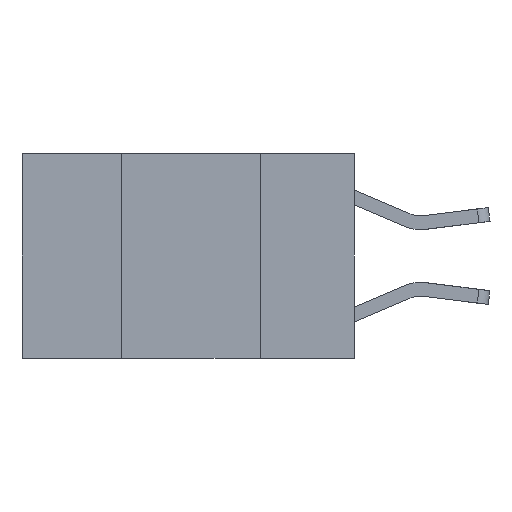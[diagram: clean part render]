
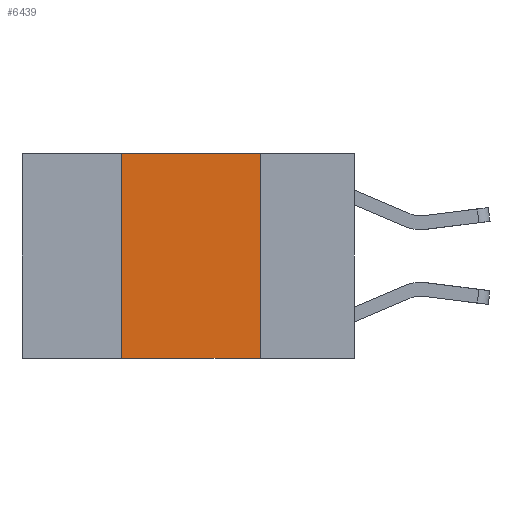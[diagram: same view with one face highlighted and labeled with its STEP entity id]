
A CAD part, left-side view. The second image highlights one B-rep face of the part: STEP entity #6439.
In plain terms, the highlighted planar face has unit normal (-1, 0, 0).
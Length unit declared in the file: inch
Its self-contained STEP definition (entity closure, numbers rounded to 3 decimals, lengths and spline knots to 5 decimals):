
#240 = LINE ( 'NONE', #5498, #8118 ) ;
#635 = CARTESIAN_POINT ( 'NONE',  ( 0., 0.6, 0. ) ) ;
#1323 = PLANE ( 'NONE',  #7634 ) ;
#2004 = CARTESIAN_POINT ( 'NONE',  ( 0., 0.42, -0.37 ) ) ;
#2282 = VERTEX_POINT ( 'NONE', #3183 ) ;
#2429 = DIRECTION ( 'NONE',  ( 0., -1., 0. ) ) ;
#2654 = VERTEX_POINT ( 'NONE', #2004 ) ;
#2915 = ORIENTED_EDGE ( 'NONE', *, *, #7851, .F. ) ;
#3114 = DIRECTION ( 'NONE',  ( 0., -1., 0. ) ) ;
#3183 = CARTESIAN_POINT ( 'NONE',  ( 0., 0.17, -0.37 ) ) ;
#3689 = VERTEX_POINT ( 'NONE', #6829 ) ;
#3702 = VECTOR ( 'NONE', #3878, 39.37008 ) ;
#3878 = DIRECTION ( 'NONE',  ( 0., 0., 1. ) ) ;
#3950 = VECTOR ( 'NONE', #4999, 39.37008 ) ;
#4228 = CARTESIAN_POINT ( 'NONE',  ( 0., 0.17, 0. ) ) ;
#4444 = CARTESIAN_POINT ( 'NONE',  ( 0., 0.17, 0. ) ) ;
#4491 = DIRECTION ( 'NONE',  ( 1., 0., 0. ) ) ;
#4704 = ORIENTED_EDGE ( 'NONE', *, *, #6842, .F. ) ;
#4999 = DIRECTION ( 'NONE',  ( 0., 0., -1. ) ) ;
#5376 = CARTESIAN_POINT ( 'NONE',  ( 0., 0.42, 0. ) ) ;
#5445 = VECTOR ( 'NONE', #3114, 39.37008 ) ;
#5498 = CARTESIAN_POINT ( 'NONE',  ( 0., 0.6, -0.37 ) ) ;
#6357 = LINE ( 'NONE', #4228, #3950 ) ;
#6439 = ADVANCED_FACE ( 'NONE', ( #6707 ), #1323, .F. ) ;
#6707 = FACE_OUTER_BOUND ( 'NONE', #9306, .T. ) ;
#6829 = CARTESIAN_POINT ( 'NONE',  ( 0., 0.42, 0. ) ) ;
#6842 = EDGE_CURVE ( 'NONE', #9177, #2282, #6357, .T. ) ;
#7332 = LINE ( 'NONE', #635, #5445 ) ;
#7634 = AXIS2_PLACEMENT_3D ( 'NONE', #8819, #4491, #9532 ) ;
#7851 = EDGE_CURVE ( 'NONE', #2654, #3689, #9478, .T. ) ;
#8118 = VECTOR ( 'NONE', #2429, 39.37008 ) ;
#8545 = ORIENTED_EDGE ( 'NONE', *, *, #9338, .F. ) ;
#8774 = ORIENTED_EDGE ( 'NONE', *, *, #9477, .T. ) ;
#8819 = CARTESIAN_POINT ( 'NONE',  ( 0., 0.6, 0. ) ) ;
#9177 = VERTEX_POINT ( 'NONE', #4444 ) ;
#9306 = EDGE_LOOP ( 'NONE', ( #4704, #8545, #2915, #8774 ) ) ;
#9338 = EDGE_CURVE ( 'NONE', #3689, #9177, #7332, .T. ) ;
#9477 = EDGE_CURVE ( 'NONE', #2654, #2282, #240, .T. ) ;
#9478 = LINE ( 'NONE', #5376, #3702 ) ;
#9532 = DIRECTION ( 'NONE',  ( 0., 0., -1. ) ) ;
